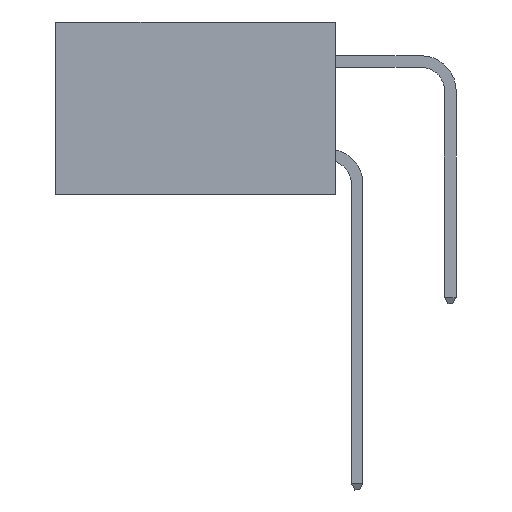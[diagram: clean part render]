
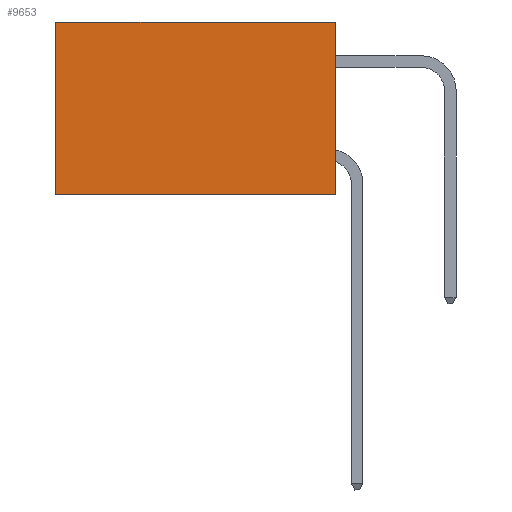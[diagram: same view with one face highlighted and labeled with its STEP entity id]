
A CAD part, left-side view. The second image highlights one B-rep face of the part: STEP entity #9653.
In plain terms, the highlighted planar face has unit normal (-1, 0, 0).
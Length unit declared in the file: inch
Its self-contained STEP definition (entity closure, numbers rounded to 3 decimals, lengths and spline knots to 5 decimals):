
#145 = LINE ( 'NONE', #1799, #10618 ) ;
#166 = CARTESIAN_POINT ( 'NONE',  ( 0.2875, 0., 0. ) ) ;
#403 = ORIENTED_EDGE ( 'NONE', *, *, #10439, .T. ) ;
#1077 = VECTOR ( 'NONE', #5541, 39.37008 ) ;
#1380 = CARTESIAN_POINT ( 'NONE',  ( 0.2875, 0., 0. ) ) ;
#1799 = CARTESIAN_POINT ( 'NONE',  ( 0.2875, 0., -0.37 ) ) ;
#2737 = DIRECTION ( 'NONE',  ( 1., 0., 0. ) ) ;
#3158 = CARTESIAN_POINT ( 'NONE',  ( 0.2875, 0.6, 0. ) ) ;
#4403 = CARTESIAN_POINT ( 'NONE',  ( 0.2875, 0.6, 0. ) ) ;
#5351 = EDGE_CURVE ( 'NONE', #13979, #13024, #145, .T. ) ;
#5541 = DIRECTION ( 'NONE',  ( 0., 0., -1. ) ) ;
#6174 = VECTOR ( 'NONE', #8251, 39.37008 ) ;
#6198 = DIRECTION ( 'NONE',  ( 0., 1., 0. ) ) ;
#6343 = VERTEX_POINT ( 'NONE', #1380 ) ;
#6449 = DIRECTION ( 'NONE',  ( 0., 1., 0. ) ) ;
#6612 = VERTEX_POINT ( 'NONE', #3158 ) ;
#6615 = ORIENTED_EDGE ( 'NONE', *, *, #5351, .F. ) ;
#6974 = ORIENTED_EDGE ( 'NONE', *, *, #12987, .T. ) ;
#7349 = AXIS2_PLACEMENT_3D ( 'NONE', #12937, #2737, #10744 ) ;
#7817 = LINE ( 'NONE', #9898, #13816 ) ;
#8251 = DIRECTION ( 'NONE',  ( 0., 0., -1. ) ) ;
#8953 = FACE_OUTER_BOUND ( 'NONE', #9970, .T. ) ;
#9581 = LINE ( 'NONE', #166, #6174 ) ;
#9620 = PLANE ( 'NONE',  #7349 ) ;
#9653 = ADVANCED_FACE ( 'NONE', ( #8953 ), #9620, .F. ) ;
#9661 = ORIENTED_EDGE ( 'NONE', *, *, #13360, .F. ) ;
#9898 = CARTESIAN_POINT ( 'NONE',  ( 0.2875, 0., 0. ) ) ;
#9970 = EDGE_LOOP ( 'NONE', ( #403, #6615, #9661, #6974 ) ) ;
#9974 = LINE ( 'NONE', #4403, #1077 ) ;
#10439 = EDGE_CURVE ( 'NONE', #6612, #13024, #9974, .T. ) ;
#10618 = VECTOR ( 'NONE', #6198, 39.37008 ) ;
#10744 = DIRECTION ( 'NONE',  ( 0., 0., -1. ) ) ;
#12192 = CARTESIAN_POINT ( 'NONE',  ( 0.2875, 0.6, -0.37 ) ) ;
#12937 = CARTESIAN_POINT ( 'NONE',  ( 0.2875, 0., 0. ) ) ;
#12987 = EDGE_CURVE ( 'NONE', #6343, #6612, #7817, .T. ) ;
#13024 = VERTEX_POINT ( 'NONE', #12192 ) ;
#13360 = EDGE_CURVE ( 'NONE', #6343, #13979, #9581, .T. ) ;
#13816 = VECTOR ( 'NONE', #6449, 39.37008 ) ;
#13908 = CARTESIAN_POINT ( 'NONE',  ( 0.2875, 0., -0.37 ) ) ;
#13979 = VERTEX_POINT ( 'NONE', #13908 ) ;
